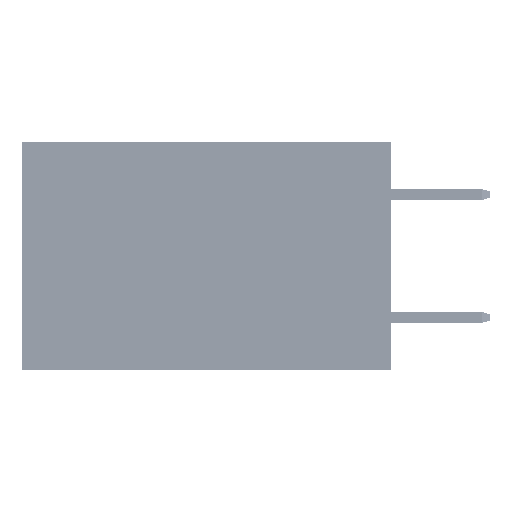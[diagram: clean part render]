
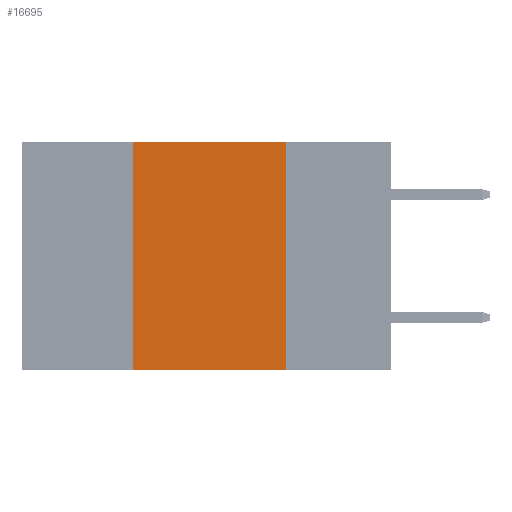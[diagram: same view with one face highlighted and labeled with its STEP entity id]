
A CAD part, left-side view. The second image highlights one B-rep face of the part: STEP entity #16695.
In plain terms, the highlighted planar face has unit normal (-1, 0, 0).
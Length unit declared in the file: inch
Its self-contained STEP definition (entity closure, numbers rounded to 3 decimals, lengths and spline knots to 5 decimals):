
#328 = VERTEX_POINT ( 'NONE', #5256 ) ;
#990 = CARTESIAN_POINT ( 'NONE',  ( 0., 0.17, 0. ) ) ;
#1258 = LINE ( 'NONE', #24040, #33996 ) ;
#2219 = ORIENTED_EDGE ( 'NONE', *, *, #37394, .T. ) ;
#2850 = EDGE_CURVE ( 'NONE', #48736, #328, #29080, .T. ) ;
#4850 = EDGE_CURVE ( 'NONE', #328, #44758, #1258, .T. ) ;
#4967 = CARTESIAN_POINT ( 'NONE',  ( 0., 0.17, 0. ) ) ;
#5256 = CARTESIAN_POINT ( 'NONE',  ( 0., 0.42, 0. ) ) ;
#7368 = ORIENTED_EDGE ( 'NONE', *, *, #41015, .F. ) ;
#8556 = CARTESIAN_POINT ( 'NONE',  ( 0., 0.42, -0.37 ) ) ;
#9364 = DIRECTION ( 'NONE',  ( 0., 0., 1. ) ) ;
#15098 = DIRECTION ( 'NONE',  ( 0., -1., 0. ) ) ;
#16695 = ADVANCED_FACE ( 'NONE', ( #36311 ), #18180, .F. ) ;
#17378 = ORIENTED_EDGE ( 'NONE', *, *, #4850, .F. ) ;
#17592 = VECTOR ( 'NONE', #26097, 39.37008 ) ;
#18180 = PLANE ( 'NONE',  #20896 ) ;
#19335 = CARTESIAN_POINT ( 'NONE',  ( 0., 0.6, -0.37 ) ) ;
#19465 = LINE ( 'NONE', #4967, #17592 ) ;
#20896 = AXIS2_PLACEMENT_3D ( 'NONE', #50309, #39834, #51954 ) ;
#24040 = CARTESIAN_POINT ( 'NONE',  ( 0., 0.6, 0. ) ) ;
#25163 = EDGE_LOOP ( 'NONE', ( #7368, #17378, #31156, #2219 ) ) ;
#25576 = CARTESIAN_POINT ( 'NONE',  ( 0., 0.42, 0. ) ) ;
#26097 = DIRECTION ( 'NONE',  ( 0., 0., -1. ) ) ;
#27985 = VERTEX_POINT ( 'NONE', #44142 ) ;
#29080 = LINE ( 'NONE', #25576, #42893 ) ;
#30012 = VECTOR ( 'NONE', #15098, 39.37008 ) ;
#31156 = ORIENTED_EDGE ( 'NONE', *, *, #2850, .F. ) ;
#33996 = VECTOR ( 'NONE', #48242, 39.37008 ) ;
#36311 = FACE_OUTER_BOUND ( 'NONE', #25163, .T. ) ;
#37394 = EDGE_CURVE ( 'NONE', #48736, #27985, #40669, .T. ) ;
#39834 = DIRECTION ( 'NONE',  ( 1., 0., 0. ) ) ;
#40669 = LINE ( 'NONE', #19335, #30012 ) ;
#41015 = EDGE_CURVE ( 'NONE', #44758, #27985, #19465, .T. ) ;
#42893 = VECTOR ( 'NONE', #9364, 39.37008 ) ;
#44142 = CARTESIAN_POINT ( 'NONE',  ( 0., 0.17, -0.37 ) ) ;
#44758 = VERTEX_POINT ( 'NONE', #990 ) ;
#48242 = DIRECTION ( 'NONE',  ( 0., -1., 0. ) ) ;
#48736 = VERTEX_POINT ( 'NONE', #8556 ) ;
#50309 = CARTESIAN_POINT ( 'NONE',  ( 0., 0.6, 0. ) ) ;
#51954 = DIRECTION ( 'NONE',  ( 0., 0., -1. ) ) ;
